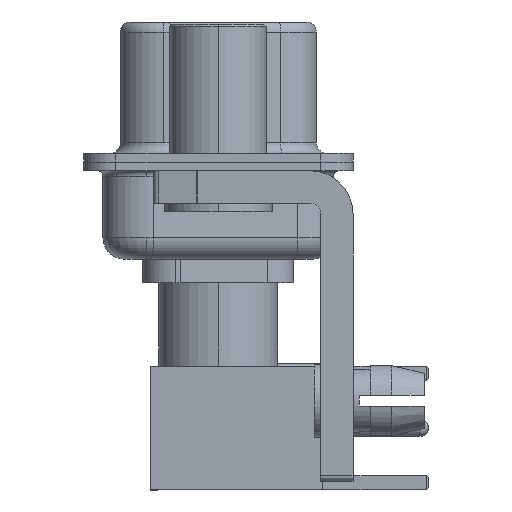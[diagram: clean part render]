
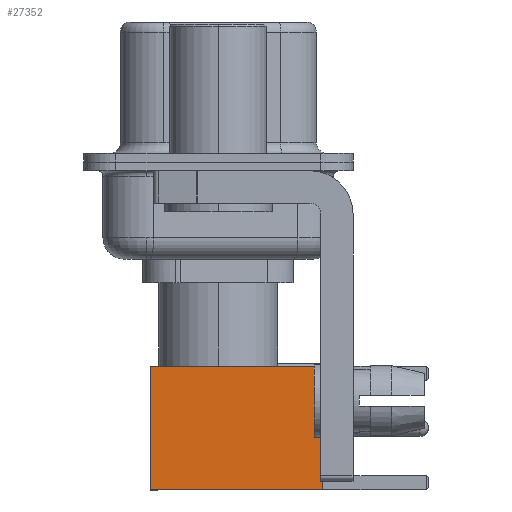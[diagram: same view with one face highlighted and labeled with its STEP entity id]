
A CAD part, left-side view. The second image highlights one B-rep face of the part: STEP entity #27352.
In plain terms, the highlighted face is planar.
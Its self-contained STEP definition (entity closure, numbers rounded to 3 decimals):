
#585 = EDGE_CURVE ( 'NONE', #7894, #1755, #11407, .T. ) ;
#605 = VECTOR ( 'NONE', #645, 1000. ) ;
#645 = DIRECTION ( 'NONE',  ( 0., 0., -1. ) ) ;
#1302 = LINE ( 'NONE', #3823, #605 ) ;
#1613 = CARTESIAN_POINT ( 'NONE',  ( 2.875, 2.875, 0. ) ) ;
#1755 = VERTEX_POINT ( 'NONE', #8158 ) ;
#2118 = EDGE_CURVE ( 'NONE', #22621, #1755, #29627, .T. ) ;
#2643 = CARTESIAN_POINT ( 'NONE',  ( 2.875, 2.875, 0. ) ) ;
#3823 = CARTESIAN_POINT ( 'NONE',  ( 2.875, 2.875, 0. ) ) ;
#6369 = CARTESIAN_POINT ( 'NONE',  ( 0., 2.875, 0. ) ) ;
#6639 = CARTESIAN_POINT ( 'NONE',  ( -2.875, 2.875, 0. ) ) ;
#6969 = VECTOR ( 'NONE', #16877, 1000. ) ;
#7894 = VERTEX_POINT ( 'NONE', #1613 ) ;
#8158 = CARTESIAN_POINT ( 'NONE',  ( -2.875, 2.875, 0. ) ) ;
#9802 = CARTESIAN_POINT ( 'NONE',  ( -2.875, 2.875, 8. ) ) ;
#11407 = LINE ( 'NONE', #6369, #32434 ) ;
#13446 = ORIENTED_EDGE ( 'NONE', *, *, #23837, .T. ) ;
#14816 = DIRECTION ( 'NONE',  ( -1., 0., 0. ) ) ;
#16877 = DIRECTION ( 'NONE',  ( 0., 0., -1. ) ) ;
#18216 = PLANE ( 'NONE',  #26912 ) ;
#18288 = CARTESIAN_POINT ( 'NONE',  ( 2.875, 2.875, 8. ) ) ;
#21357 = FACE_OUTER_BOUND ( 'NONE', #30497, .T. ) ;
#22029 = VERTEX_POINT ( 'NONE', #18288 ) ;
#22177 = LINE ( 'NONE', #27560, #30618 ) ;
#22621 = VERTEX_POINT ( 'NONE', #9802 ) ;
#23837 = EDGE_CURVE ( 'NONE', #22029, #7894, #1302, .T. ) ;
#26080 = ORIENTED_EDGE ( 'NONE', *, *, #27495, .F. ) ;
#26912 = AXIS2_PLACEMENT_3D ( 'NONE', #2643, #31590, #30659 ) ;
#27352 = ADVANCED_FACE ( 'NONE', ( #21357 ), #18216, .T. ) ;
#27495 = EDGE_CURVE ( 'NONE', #22029, #22621, #22177, .T. ) ;
#27560 = CARTESIAN_POINT ( 'NONE',  ( 0., 2.875, 8. ) ) ;
#27608 = ORIENTED_EDGE ( 'NONE', *, *, #585, .T. ) ;
#27932 = ORIENTED_EDGE ( 'NONE', *, *, #2118, .F. ) ;
#29627 = LINE ( 'NONE', #6639, #6969 ) ;
#30158 = DIRECTION ( 'NONE',  ( -1., 0., 0. ) ) ;
#30497 = EDGE_LOOP ( 'NONE', ( #13446, #27608, #27932, #26080 ) ) ;
#30618 = VECTOR ( 'NONE', #14816, 1000. ) ;
#30659 = DIRECTION ( 'NONE',  ( 0., 0., 1. ) ) ;
#31590 = DIRECTION ( 'NONE',  ( 0., 1., 0. ) ) ;
#32434 = VECTOR ( 'NONE', #30158, 1000. ) ;
